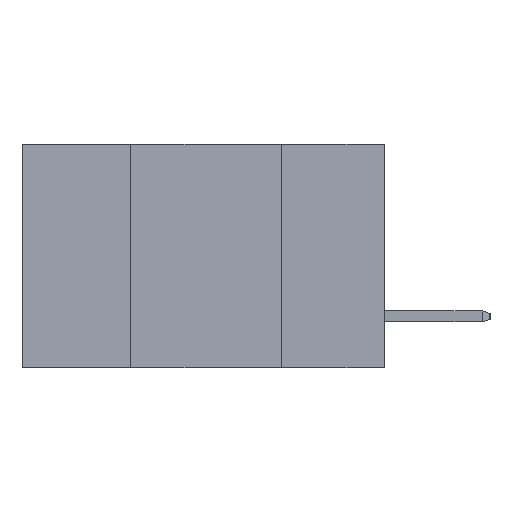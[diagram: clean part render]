
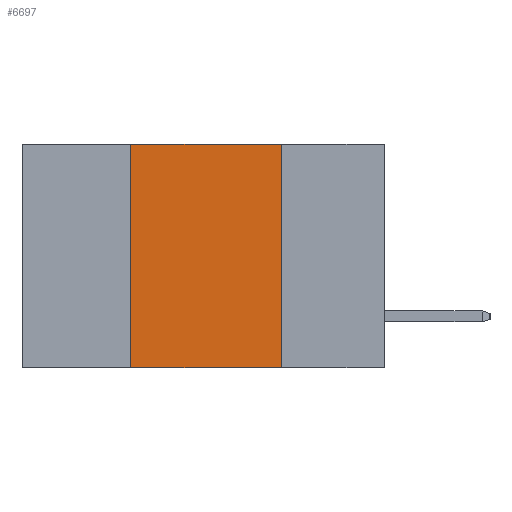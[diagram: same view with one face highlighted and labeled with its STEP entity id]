
A CAD part, left-side view. The second image highlights one B-rep face of the part: STEP entity #6697.
In plain terms, the highlighted planar face has unit normal (-1, 0, 0).
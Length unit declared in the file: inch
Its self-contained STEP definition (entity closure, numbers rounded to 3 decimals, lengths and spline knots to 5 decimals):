
#166 = DIRECTION ( 'NONE',  ( 1., 0., 0. ) ) ;
#285 = VERTEX_POINT ( 'NONE', #13322 ) ;
#576 = AXIS2_PLACEMENT_3D ( 'NONE', #12421, #166, #14495 ) ;
#2443 = VECTOR ( 'NONE', #26271, 39.37008 ) ;
#2691 = ORIENTED_EDGE ( 'NONE', *, *, #16807, .F. ) ;
#4482 = VECTOR ( 'NONE', #21169, 39.37008 ) ;
#4651 = LINE ( 'NONE', #6661, #25836 ) ;
#5433 = CARTESIAN_POINT ( 'NONE',  ( 0., 0.17, -0.37 ) ) ;
#5854 = CARTESIAN_POINT ( 'NONE',  ( 0., 0.42, -0.37 ) ) ;
#6661 = CARTESIAN_POINT ( 'NONE',  ( 0., 0.6, -0.37 ) ) ;
#6697 = ADVANCED_FACE ( 'NONE', ( #22522 ), #22695, .F. ) ;
#6989 = VERTEX_POINT ( 'NONE', #5433 ) ;
#8464 = VECTOR ( 'NONE', #14430, 39.37008 ) ;
#8480 = EDGE_CURVE ( 'NONE', #20075, #6989, #4651, .T. ) ;
#10344 = CARTESIAN_POINT ( 'NONE',  ( 0., 0.42, 0. ) ) ;
#12421 = CARTESIAN_POINT ( 'NONE',  ( 0., 0.6, 0. ) ) ;
#12701 = LINE ( 'NONE', #24280, #2443 ) ;
#13322 = CARTESIAN_POINT ( 'NONE',  ( 0., 0.17, 0. ) ) ;
#14039 = EDGE_CURVE ( 'NONE', #20075, #20102, #24895, .T. ) ;
#14430 = DIRECTION ( 'NONE',  ( 0., 0., 1. ) ) ;
#14495 = DIRECTION ( 'NONE',  ( 0., 0., -1. ) ) ;
#15101 = LINE ( 'NONE', #23039, #4482 ) ;
#16807 = EDGE_CURVE ( 'NONE', #20102, #285, #15101, .T. ) ;
#18156 = EDGE_LOOP ( 'NONE', ( #21109, #2691, #18636, #25871 ) ) ;
#18636 = ORIENTED_EDGE ( 'NONE', *, *, #14039, .F. ) ;
#19085 = DIRECTION ( 'NONE',  ( 0., -1., 0. ) ) ;
#19611 = EDGE_CURVE ( 'NONE', #285, #6989, #12701, .T. ) ;
#20075 = VERTEX_POINT ( 'NONE', #5854 ) ;
#20102 = VERTEX_POINT ( 'NONE', #20417 ) ;
#20417 = CARTESIAN_POINT ( 'NONE',  ( 0., 0.42, 0. ) ) ;
#21109 = ORIENTED_EDGE ( 'NONE', *, *, #19611, .F. ) ;
#21169 = DIRECTION ( 'NONE',  ( 0., -1., 0. ) ) ;
#22522 = FACE_OUTER_BOUND ( 'NONE', #18156, .T. ) ;
#22695 = PLANE ( 'NONE',  #576 ) ;
#23039 = CARTESIAN_POINT ( 'NONE',  ( 0., 0.6, 0. ) ) ;
#24280 = CARTESIAN_POINT ( 'NONE',  ( 0., 0.17, 0. ) ) ;
#24895 = LINE ( 'NONE', #10344, #8464 ) ;
#25836 = VECTOR ( 'NONE', #19085, 39.37008 ) ;
#25871 = ORIENTED_EDGE ( 'NONE', *, *, #8480, .T. ) ;
#26271 = DIRECTION ( 'NONE',  ( 0., 0., -1. ) ) ;
